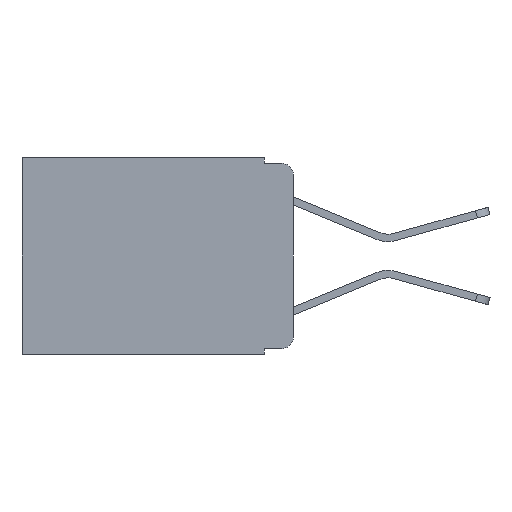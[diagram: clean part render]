
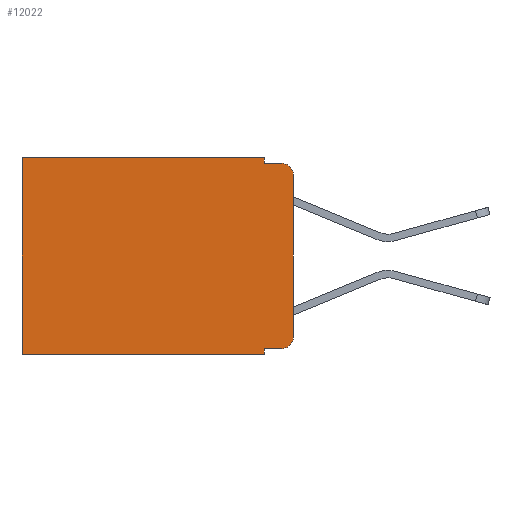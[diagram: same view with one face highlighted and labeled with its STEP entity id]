
A CAD part, left-side view. The second image highlights one B-rep face of the part: STEP entity #12022.
In plain terms, the highlighted planar face has unit normal (-1, 0, 0).
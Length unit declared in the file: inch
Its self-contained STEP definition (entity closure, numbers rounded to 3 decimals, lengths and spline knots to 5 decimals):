
#593 = DIRECTION ( 'NONE',  ( 0., -1., 0. ) ) ;
#604 = VERTEX_POINT ( 'NONE', #16185 ) ;
#644 = EDGE_CURVE ( 'NONE', #23045, #9742, #21502, .T. ) ;
#672 = CARTESIAN_POINT ( 'NONE',  ( 0.298, 0.051, -0.333 ) ) ;
#729 = DIRECTION ( 'NONE',  ( 0., -1., 0. ) ) ;
#2536 = LINE ( 'NONE', #3107, #7231 ) ;
#2803 = CARTESIAN_POINT ( 'NONE',  ( 0.298, 0., -0.343 ) ) ;
#3029 = EDGE_LOOP ( 'NONE', ( #9835, #20863, #18853, #15808, #14154, #19881, #16108, #11106, #14147, #6915 ) ) ;
#3107 = CARTESIAN_POINT ( 'NONE',  ( 0.298, 0.473, 0. ) ) ;
#3671 = VECTOR ( 'NONE', #729, 39.37008 ) ;
#3678 = FACE_OUTER_BOUND ( 'NONE', #3029, .T. ) ;
#4113 = VERTEX_POINT ( 'NONE', #17832 ) ;
#4188 = VERTEX_POINT ( 'NONE', #16181 ) ;
#4618 = EDGE_CURVE ( 'NONE', #16426, #604, #11679, .T. ) ;
#4654 = EDGE_CURVE ( 'NONE', #19563, #4113, #5848, .T. ) ;
#4685 = DIRECTION ( 'NONE',  ( 0., 0., -1. ) ) ;
#5483 = VECTOR ( 'NONE', #21367, 39.37008 ) ;
#5848 = LINE ( 'NONE', #672, #20157 ) ;
#6331 = VECTOR ( 'NONE', #19211, 39.37008 ) ;
#6653 = PLANE ( 'NONE',  #13122 ) ;
#6706 = DIRECTION ( 'NONE',  ( 0., 0., -1. ) ) ;
#6730 = CARTESIAN_POINT ( 'NONE',  ( 0.298, 0., -0.03 ) ) ;
#6915 = ORIENTED_EDGE ( 'NONE', *, *, #10670, .T. ) ;
#7231 = VECTOR ( 'NONE', #6706, 39.37008 ) ;
#8110 = CIRCLE ( 'NONE', #15276, 0.02 ) ;
#9479 = CARTESIAN_POINT ( 'NONE',  ( 0.298, 0.051, -0.343 ) ) ;
#9741 = DIRECTION ( 'NONE',  ( 0., 0., -1. ) ) ;
#9742 = VERTEX_POINT ( 'NONE', #10259 ) ;
#9835 = ORIENTED_EDGE ( 'NONE', *, *, #18917, .F. ) ;
#10030 = CARTESIAN_POINT ( 'NONE',  ( 0.298, 0.051, -0.01 ) ) ;
#10259 = CARTESIAN_POINT ( 'NONE',  ( 0.298, 0.473, 0. ) ) ;
#10450 = LINE ( 'NONE', #19824, #5483 ) ;
#10454 = LINE ( 'NONE', #13608, #19230 ) ;
#10543 = EDGE_CURVE ( 'NONE', #19563, #10994, #10454, .T. ) ;
#10670 = EDGE_CURVE ( 'NONE', #4113, #4188, #8110, .T. ) ;
#10785 = EDGE_CURVE ( 'NONE', #9742, #11831, #2536, .T. ) ;
#10994 = VERTEX_POINT ( 'NONE', #9479 ) ;
#11106 = ORIENTED_EDGE ( 'NONE', *, *, #10543, .F. ) ;
#11679 = CIRCLE ( 'NONE', #15489, 0.02 ) ;
#11831 = VERTEX_POINT ( 'NONE', #21257 ) ;
#12022 = ADVANCED_FACE ( 'NONE', ( #3678 ), #6653, .F. ) ;
#12032 = DIRECTION ( 'NONE',  ( 0., 0., -1. ) ) ;
#12363 = DIRECTION ( 'NONE',  ( 0., 0., -1. ) ) ;
#12472 = CARTESIAN_POINT ( 'NONE',  ( 0.298, 0., 0. ) ) ;
#13122 = AXIS2_PLACEMENT_3D ( 'NONE', #12472, #16192, #4685 ) ;
#13203 = CARTESIAN_POINT ( 'NONE',  ( 0.298, 0.051, -0.01 ) ) ;
#13345 = EDGE_CURVE ( 'NONE', #10994, #11831, #20555, .T. ) ;
#13608 = CARTESIAN_POINT ( 'NONE',  ( 0.298, 0.051, 0. ) ) ;
#13617 = VERTEX_POINT ( 'NONE', #13203 ) ;
#13746 = CARTESIAN_POINT ( 'NONE',  ( 0.298, 0.02, -0.03 ) ) ;
#14147 = ORIENTED_EDGE ( 'NONE', *, *, #4654, .T. ) ;
#14154 = ORIENTED_EDGE ( 'NONE', *, *, #644, .T. ) ;
#15276 = AXIS2_PLACEMENT_3D ( 'NONE', #18143, #16090, #12363 ) ;
#15437 = VECTOR ( 'NONE', #12032, 39.37008 ) ;
#15489 = AXIS2_PLACEMENT_3D ( 'NONE', #13746, #23100, #9741 ) ;
#15808 = ORIENTED_EDGE ( 'NONE', *, *, #22019, .F. ) ;
#16090 = DIRECTION ( 'NONE',  ( -1., 0., 0. ) ) ;
#16108 = ORIENTED_EDGE ( 'NONE', *, *, #13345, .F. ) ;
#16109 = DIRECTION ( 'NONE',  ( 0., 1., 0. ) ) ;
#16181 = CARTESIAN_POINT ( 'NONE',  ( 0.298, 0., -0.313 ) ) ;
#16185 = CARTESIAN_POINT ( 'NONE',  ( 0.298, 0.02, -0.01 ) ) ;
#16192 = DIRECTION ( 'NONE',  ( 1., 0., 0. ) ) ;
#16426 = VERTEX_POINT ( 'NONE', #6730 ) ;
#16822 = CARTESIAN_POINT ( 'NONE',  ( 0.298, 0., 0. ) ) ;
#17832 = CARTESIAN_POINT ( 'NONE',  ( 0.298, 0.02, -0.333 ) ) ;
#17930 = VECTOR ( 'NONE', #16109, 39.37008 ) ;
#17995 = LINE ( 'NONE', #10030, #3671 ) ;
#18068 = CARTESIAN_POINT ( 'NONE',  ( 0.298, 0.051, 0. ) ) ;
#18143 = CARTESIAN_POINT ( 'NONE',  ( 0.298, 0.02, -0.313 ) ) ;
#18853 = ORIENTED_EDGE ( 'NONE', *, *, #20858, .F. ) ;
#18917 = EDGE_CURVE ( 'NONE', #16426, #4188, #19245, .T. ) ;
#19101 = CARTESIAN_POINT ( 'NONE',  ( 0.298, 0.051, -0.333 ) ) ;
#19211 = DIRECTION ( 'NONE',  ( 0., 1., 0. ) ) ;
#19230 = VECTOR ( 'NONE', #19303, 39.37008 ) ;
#19245 = LINE ( 'NONE', #23201, #15437 ) ;
#19303 = DIRECTION ( 'NONE',  ( 0., 0., -1. ) ) ;
#19563 = VERTEX_POINT ( 'NONE', #19101 ) ;
#19824 = CARTESIAN_POINT ( 'NONE',  ( 0.298, 0.051, 0. ) ) ;
#19881 = ORIENTED_EDGE ( 'NONE', *, *, #10785, .T. ) ;
#20157 = VECTOR ( 'NONE', #593, 39.37008 ) ;
#20555 = LINE ( 'NONE', #2803, #17930 ) ;
#20858 = EDGE_CURVE ( 'NONE', #13617, #604, #17995, .T. ) ;
#20863 = ORIENTED_EDGE ( 'NONE', *, *, #4618, .T. ) ;
#21257 = CARTESIAN_POINT ( 'NONE',  ( 0.298, 0.473, -0.343 ) ) ;
#21367 = DIRECTION ( 'NONE',  ( 0., 0., -1. ) ) ;
#21502 = LINE ( 'NONE', #16822, #6331 ) ;
#22019 = EDGE_CURVE ( 'NONE', #23045, #13617, #10450, .T. ) ;
#23045 = VERTEX_POINT ( 'NONE', #18068 ) ;
#23100 = DIRECTION ( 'NONE',  ( -1., 0., 0. ) ) ;
#23201 = CARTESIAN_POINT ( 'NONE',  ( 0.298, 0., 0. ) ) ;
